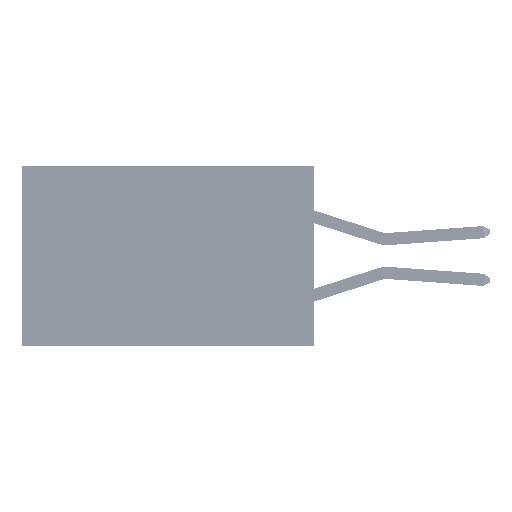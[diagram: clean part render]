
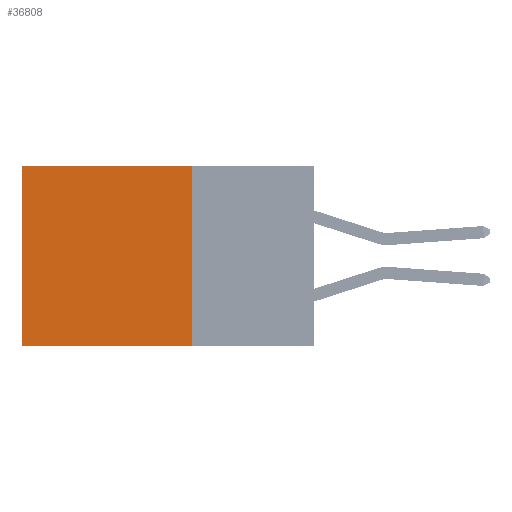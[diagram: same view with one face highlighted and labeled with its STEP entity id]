
A CAD part, left-side view. The second image highlights one B-rep face of the part: STEP entity #36808.
In plain terms, the highlighted planar face has unit normal (-1, 0, 0).
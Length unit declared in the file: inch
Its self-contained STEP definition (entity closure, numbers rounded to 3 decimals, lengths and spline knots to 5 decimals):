
#1584 = EDGE_CURVE ( 'NONE', #7743, #2541, #18990, .T. ) ;
#1842 = FACE_OUTER_BOUND ( 'NONE', #11694, .T. ) ;
#2541 = VERTEX_POINT ( 'NONE', #15444 ) ;
#3318 = AXIS2_PLACEMENT_3D ( 'NONE', #39601, #32711, #26326 ) ;
#5529 = CARTESIAN_POINT ( 'NONE',  ( 0.2875, 0.25, -0.37 ) ) ;
#5978 = DIRECTION ( 'NONE',  ( 0., 1., 0. ) ) ;
#6417 = LINE ( 'NONE', #5529, #22858 ) ;
#6542 = ORIENTED_EDGE ( 'NONE', *, *, #41058, .T. ) ;
#7445 = ORIENTED_EDGE ( 'NONE', *, *, #34294, .F. ) ;
#7743 = VERTEX_POINT ( 'NONE', #8421 ) ;
#8421 = CARTESIAN_POINT ( 'NONE',  ( 0.2875, 0.25, 0. ) ) ;
#10527 = CARTESIAN_POINT ( 'NONE',  ( 0.2875, 0.6, 0. ) ) ;
#11445 = DIRECTION ( 'NONE',  ( 0., 0., -1. ) ) ;
#11694 = EDGE_LOOP ( 'NONE', ( #18820, #7445, #15349, #6542 ) ) ;
#15349 = ORIENTED_EDGE ( 'NONE', *, *, #1584, .F. ) ;
#15444 = CARTESIAN_POINT ( 'NONE',  ( 0.2875, 0.25, -0.37 ) ) ;
#15806 = PLANE ( 'NONE',  #3318 ) ;
#18820 = ORIENTED_EDGE ( 'NONE', *, *, #21153, .T. ) ;
#18990 = LINE ( 'NONE', #32223, #40272 ) ;
#21153 = EDGE_CURVE ( 'NONE', #22737, #43132, #36608, .T. ) ;
#22737 = VERTEX_POINT ( 'NONE', #10527 ) ;
#22858 = VECTOR ( 'NONE', #5978, 39.37008 ) ;
#26326 = DIRECTION ( 'NONE',  ( 0., 0., -1. ) ) ;
#27000 = VECTOR ( 'NONE', #43260, 39.37008 ) ;
#27360 = CARTESIAN_POINT ( 'NONE',  ( 0.2875, 0.6, -0.37 ) ) ;
#27654 = DIRECTION ( 'NONE',  ( 0., 1., 0. ) ) ;
#29967 = CARTESIAN_POINT ( 'NONE',  ( 0.2875, 0.6, 0. ) ) ;
#31080 = LINE ( 'NONE', #40966, #36908 ) ;
#32223 = CARTESIAN_POINT ( 'NONE',  ( 0.2875, 0.25, 0. ) ) ;
#32711 = DIRECTION ( 'NONE',  ( 1., 0., 0. ) ) ;
#34294 = EDGE_CURVE ( 'NONE', #2541, #43132, #6417, .T. ) ;
#36608 = LINE ( 'NONE', #29967, #27000 ) ;
#36808 = ADVANCED_FACE ( 'NONE', ( #1842 ), #15806, .F. ) ;
#36908 = VECTOR ( 'NONE', #27654, 39.37008 ) ;
#39601 = CARTESIAN_POINT ( 'NONE',  ( 0.2875, 0.25, 0. ) ) ;
#40272 = VECTOR ( 'NONE', #11445, 39.37008 ) ;
#40966 = CARTESIAN_POINT ( 'NONE',  ( 0.2875, 0.25, 0. ) ) ;
#41058 = EDGE_CURVE ( 'NONE', #7743, #22737, #31080, .T. ) ;
#43132 = VERTEX_POINT ( 'NONE', #27360 ) ;
#43260 = DIRECTION ( 'NONE',  ( 0., 0., -1. ) ) ;
